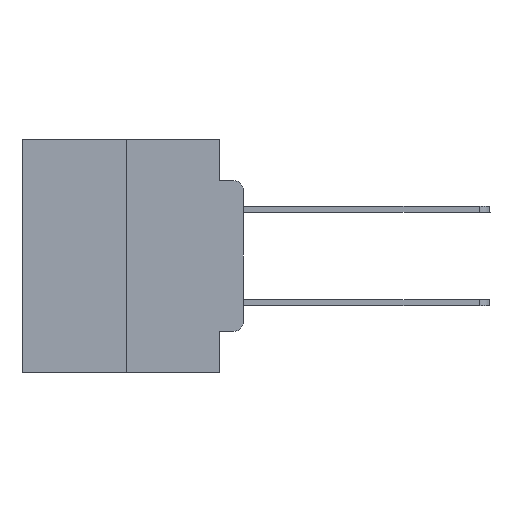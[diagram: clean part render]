
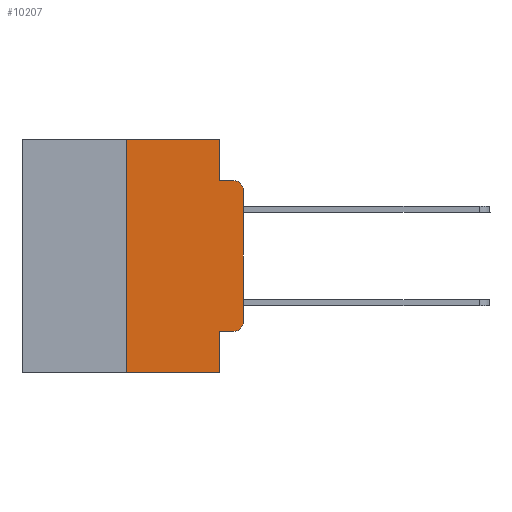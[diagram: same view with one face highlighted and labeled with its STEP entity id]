
A CAD part, left-side view. The second image highlights one B-rep face of the part: STEP entity #10207.
In plain terms, the highlighted planar face has unit normal (-1, 0, 0).
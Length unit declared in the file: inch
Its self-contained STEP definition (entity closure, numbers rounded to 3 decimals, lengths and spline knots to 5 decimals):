
#286 = LINE ( 'NONE', #21679, #16494 ) ;
#438 = CARTESIAN_POINT ( 'NONE',  ( 0., 0.25, -0.5 ) ) ;
#843 = CARTESIAN_POINT ( 'NONE',  ( 0., 0., -0.1085 ) ) ;
#1480 = EDGE_CURVE ( 'NONE', #5848, #21335, #5516, .T. ) ;
#2174 = CARTESIAN_POINT ( 'NONE',  ( 0., 0.051, -0.4115 ) ) ;
#2222 = DIRECTION ( 'NONE',  ( 0., -1., 0. ) ) ;
#2456 = EDGE_CURVE ( 'NONE', #3170, #17182, #5781, .T. ) ;
#2482 = CARTESIAN_POINT ( 'NONE',  ( 0., 0.473, 0. ) ) ;
#2596 = CARTESIAN_POINT ( 'NONE',  ( 0., 0.051, 0. ) ) ;
#3111 = CARTESIAN_POINT ( 'NONE',  ( 0., 0.051, -0.0885 ) ) ;
#3170 = VERTEX_POINT ( 'NONE', #19500 ) ;
#3992 = VERTEX_POINT ( 'NONE', #14736 ) ;
#4190 = DIRECTION ( 'NONE',  ( 0., 0., 1. ) ) ;
#4378 = AXIS2_PLACEMENT_3D ( 'NONE', #17763, #24234, #7240 ) ;
#4682 = LINE ( 'NONE', #17110, #8987 ) ;
#4711 = DIRECTION ( 'NONE',  ( 0., 0., -1. ) ) ;
#4842 = EDGE_CURVE ( 'NONE', #5800, #26669, #286, .T. ) ;
#4966 = EDGE_CURVE ( 'NONE', #17182, #12714, #10556, .T. ) ;
#5305 = ORIENTED_EDGE ( 'NONE', *, *, #20501, .T. ) ;
#5380 = VERTEX_POINT ( 'NONE', #11911 ) ;
#5516 = LINE ( 'NONE', #2596, #10801 ) ;
#5528 = EDGE_LOOP ( 'NONE', ( #27142, #19572, #11500, #14619, #5627, #17927, #18754, #24552, #12095, #5305 ) ) ;
#5627 = ORIENTED_EDGE ( 'NONE', *, *, #10903, .F. ) ;
#5781 = LINE ( 'NONE', #8511, #25592 ) ;
#5800 = VERTEX_POINT ( 'NONE', #9659 ) ;
#5848 = VERTEX_POINT ( 'NONE', #26804 ) ;
#6228 = LINE ( 'NONE', #2174, #7226 ) ;
#6287 = CARTESIAN_POINT ( 'NONE',  ( 0., 0.02, -0.1085 ) ) ;
#6680 = DIRECTION ( 'NONE',  ( 0., -1., 0. ) ) ;
#6753 = CARTESIAN_POINT ( 'NONE',  ( 0., 0.02, -0.3915 ) ) ;
#6852 = DIRECTION ( 'NONE',  ( -1., 0., 0. ) ) ;
#7022 = DIRECTION ( 'NONE',  ( 0., 0., -1. ) ) ;
#7226 = VECTOR ( 'NONE', #15556, 39.37008 ) ;
#7240 = DIRECTION ( 'NONE',  ( 0., 0., -1. ) ) ;
#7246 = VECTOR ( 'NONE', #2222, 39.37008 ) ;
#7749 = AXIS2_PLACEMENT_3D ( 'NONE', #6753, #6852, #21487 ) ;
#8511 = CARTESIAN_POINT ( 'NONE',  ( 0., 0., 0. ) ) ;
#8690 = DIRECTION ( 'NONE',  ( 0., 0., -1. ) ) ;
#8987 = VECTOR ( 'NONE', #6680, 39.37008 ) ;
#9492 = VERTEX_POINT ( 'NONE', #438 ) ;
#9659 = CARTESIAN_POINT ( 'NONE',  ( 0., 0.051, -0.4115 ) ) ;
#10207 = ADVANCED_FACE ( 'NONE', ( #12933 ), #24053, .F. ) ;
#10556 = CIRCLE ( 'NONE', #14250, 0.02 ) ;
#10801 = VECTOR ( 'NONE', #7022, 39.37008 ) ;
#10880 = DIRECTION ( 'NONE',  ( 0., -1., 0. ) ) ;
#10903 = EDGE_CURVE ( 'NONE', #3992, #5848, #17782, .T. ) ;
#11500 = ORIENTED_EDGE ( 'NONE', *, *, #14554, .F. ) ;
#11911 = CARTESIAN_POINT ( 'NONE',  ( 0., 0.02, -0.4115 ) ) ;
#12095 = ORIENTED_EDGE ( 'NONE', *, *, #17165, .T. ) ;
#12714 = VERTEX_POINT ( 'NONE', #16573 ) ;
#12933 = FACE_OUTER_BOUND ( 'NONE', #5528, .T. ) ;
#13114 = CARTESIAN_POINT ( 'NONE',  ( 0., 0.473, -0.5 ) ) ;
#14250 = AXIS2_PLACEMENT_3D ( 'NONE', #6287, #23554, #8690 ) ;
#14469 = VECTOR ( 'NONE', #10880, 39.37008 ) ;
#14554 = EDGE_CURVE ( 'NONE', #21335, #12714, #4682, .T. ) ;
#14619 = ORIENTED_EDGE ( 'NONE', *, *, #1480, .F. ) ;
#14736 = CARTESIAN_POINT ( 'NONE',  ( 0., 0.25, 0. ) ) ;
#14797 = DIRECTION ( 'NONE',  ( 0., 0., 1. ) ) ;
#14842 = CARTESIAN_POINT ( 'NONE',  ( 0., 0.25, 0. ) ) ;
#14947 = LINE ( 'NONE', #14842, #23184 ) ;
#15556 = DIRECTION ( 'NONE',  ( 0., -1., 0. ) ) ;
#16037 = EDGE_CURVE ( 'NONE', #9492, #26669, #17162, .T. ) ;
#16494 = VECTOR ( 'NONE', #4711, 39.37008 ) ;
#16573 = CARTESIAN_POINT ( 'NONE',  ( 0., 0.02, -0.0885 ) ) ;
#17110 = CARTESIAN_POINT ( 'NONE',  ( 0., 0.051, -0.0885 ) ) ;
#17162 = LINE ( 'NONE', #13114, #7246 ) ;
#17165 = EDGE_CURVE ( 'NONE', #5800, #5380, #6228, .T. ) ;
#17182 = VERTEX_POINT ( 'NONE', #843 ) ;
#17763 = CARTESIAN_POINT ( 'NONE',  ( 0., 0.473, 0. ) ) ;
#17782 = LINE ( 'NONE', #2482, #14469 ) ;
#17927 = ORIENTED_EDGE ( 'NONE', *, *, #27029, .F. ) ;
#18754 = ORIENTED_EDGE ( 'NONE', *, *, #16037, .T. ) ;
#19500 = CARTESIAN_POINT ( 'NONE',  ( 0., 0., -0.3915 ) ) ;
#19572 = ORIENTED_EDGE ( 'NONE', *, *, #4966, .T. ) ;
#19855 = CIRCLE ( 'NONE', #7749, 0.02 ) ;
#20501 = EDGE_CURVE ( 'NONE', #5380, #3170, #19855, .T. ) ;
#21335 = VERTEX_POINT ( 'NONE', #3111 ) ;
#21487 = DIRECTION ( 'NONE',  ( 0., 0., -1. ) ) ;
#21679 = CARTESIAN_POINT ( 'NONE',  ( 0., 0.051, 0. ) ) ;
#23184 = VECTOR ( 'NONE', #4190, 39.37008 ) ;
#23554 = DIRECTION ( 'NONE',  ( -1., 0., 0. ) ) ;
#24053 = PLANE ( 'NONE',  #4378 ) ;
#24128 = CARTESIAN_POINT ( 'NONE',  ( 0., 0.051, -0.5 ) ) ;
#24234 = DIRECTION ( 'NONE',  ( 1., 0., 0. ) ) ;
#24552 = ORIENTED_EDGE ( 'NONE', *, *, #4842, .F. ) ;
#25592 = VECTOR ( 'NONE', #14797, 39.37008 ) ;
#26669 = VERTEX_POINT ( 'NONE', #24128 ) ;
#26804 = CARTESIAN_POINT ( 'NONE',  ( 0., 0.051, 0. ) ) ;
#27029 = EDGE_CURVE ( 'NONE', #9492, #3992, #14947, .T. ) ;
#27142 = ORIENTED_EDGE ( 'NONE', *, *, #2456, .T. ) ;
